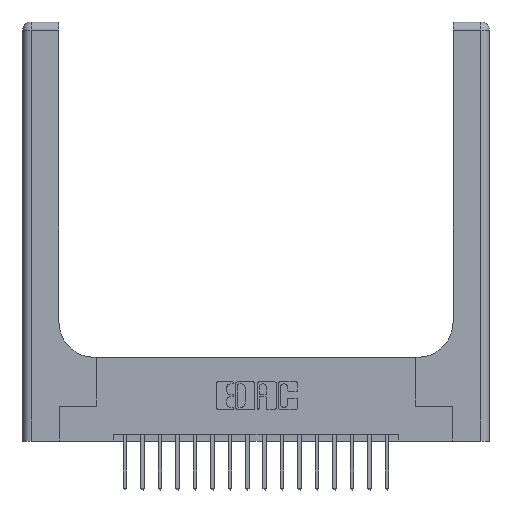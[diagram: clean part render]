
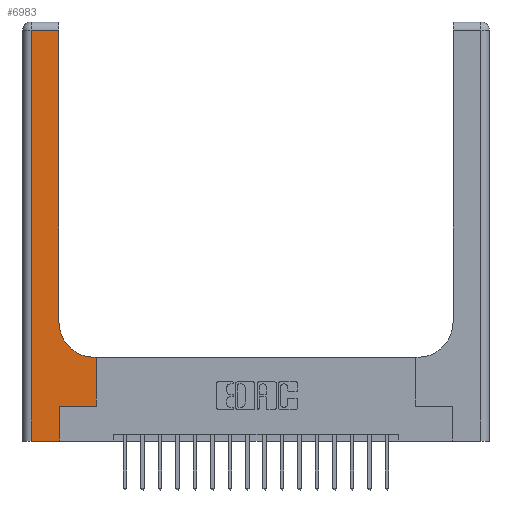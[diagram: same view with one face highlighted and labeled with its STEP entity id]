
A CAD part, top view. The second image highlights one B-rep face of the part: STEP entity #6983.
In plain terms, the highlighted planar face has unit normal (0, 0, 1).
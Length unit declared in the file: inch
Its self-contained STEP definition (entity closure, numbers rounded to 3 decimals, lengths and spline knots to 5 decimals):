
#65 = CARTESIAN_POINT ( 'NONE',  ( 0.26, 3., 0.37 ) ) ;
#98 = CARTESIAN_POINT ( 'NONE',  ( 0., 0., 0.37 ) ) ;
#191 = FACE_OUTER_BOUND ( 'NONE', #6634, .T. ) ;
#386 = CIRCLE ( 'NONE', #13804, 0.25 ) ;
#973 = VERTEX_POINT ( 'NONE', #6647 ) ;
#1305 = LINE ( 'NONE', #98, #8754 ) ;
#1519 = DIRECTION ( 'NONE',  ( 1., 0., 0. ) ) ;
#1708 = EDGE_CURVE ( 'NONE', #2682, #4155, #1305, .T. ) ;
#2682 = VERTEX_POINT ( 'NONE', #3264 ) ;
#2894 = CARTESIAN_POINT ( 'NONE',  ( 0.06, 3., 0.37 ) ) ;
#3031 = EDGE_CURVE ( 'NONE', #9360, #16881, #8223, .T. ) ;
#3187 = ORIENTED_EDGE ( 'NONE', *, *, #3360, .T. ) ;
#3260 = DIRECTION ( 'NONE',  ( 0., 0., -1. ) ) ;
#3264 = CARTESIAN_POINT ( 'NONE',  ( 0.06, 0., 0.37 ) ) ;
#3360 = EDGE_CURVE ( 'NONE', #17764, #8824, #12852, .T. ) ;
#3562 = VECTOR ( 'NONE', #6633, 39.37008 ) ;
#3802 = DIRECTION ( 'NONE',  ( 0., 1., 0. ) ) ;
#4155 = VERTEX_POINT ( 'NONE', #12005 ) ;
#4251 = DIRECTION ( 'NONE',  ( 0., 1., 0. ) ) ;
#4447 = EDGE_CURVE ( 'NONE', #4657, #17764, #12555, .T. ) ;
#4657 = VERTEX_POINT ( 'NONE', #13719 ) ;
#4870 = CARTESIAN_POINT ( 'NONE',  ( 0.51, 0.6, 0.37 ) ) ;
#4910 = DIRECTION ( 'NONE',  ( 0., 0., -1. ) ) ;
#5095 = LINE ( 'NONE', #8159, #12071 ) ;
#5936 = DIRECTION ( 'NONE',  ( 0., -1., 0. ) ) ;
#6104 = ORIENTED_EDGE ( 'NONE', *, *, #14994, .T. ) ;
#6308 = VERTEX_POINT ( 'NONE', #14318 ) ;
#6425 = CARTESIAN_POINT ( 'NONE',  ( 0.26, 2.94, 0.37 ) ) ;
#6633 = DIRECTION ( 'NONE',  ( -1., 0., 0. ) ) ;
#6634 = EDGE_LOOP ( 'NONE', ( #16386, #18016, #6104, #8862, #9578, #8550, #11908, #3187, #15459 ) ) ;
#6647 = CARTESIAN_POINT ( 'NONE',  ( 0.06, 2.94, 0.37 ) ) ;
#6983 = ADVANCED_FACE ( 'NONE', ( #191 ), #16472, .F. ) ;
#7491 = LINE ( 'NONE', #17664, #16979 ) ;
#7697 = DIRECTION ( 'NONE',  ( 0., 1., 0. ) ) ;
#8159 = CARTESIAN_POINT ( 'NONE',  ( 0.265, 0., 0.37 ) ) ;
#8223 = LINE ( 'NONE', #65, #11020 ) ;
#8550 = ORIENTED_EDGE ( 'NONE', *, *, #14991, .T. ) ;
#8754 = VECTOR ( 'NONE', #17756, 39.37008 ) ;
#8824 = VERTEX_POINT ( 'NONE', #4870 ) ;
#8862 = ORIENTED_EDGE ( 'NONE', *, *, #1708, .T. ) ;
#9360 = VERTEX_POINT ( 'NONE', #9566 ) ;
#9566 = CARTESIAN_POINT ( 'NONE',  ( 0.26, 0.85, 0.37 ) ) ;
#9578 = ORIENTED_EDGE ( 'NONE', *, *, #16562, .T. ) ;
#10056 = VECTOR ( 'NONE', #5936, 39.37008 ) ;
#10480 = VECTOR ( 'NONE', #4251, 39.37008 ) ;
#11020 = VECTOR ( 'NONE', #7697, 39.37008 ) ;
#11908 = ORIENTED_EDGE ( 'NONE', *, *, #4447, .T. ) ;
#12005 = CARTESIAN_POINT ( 'NONE',  ( 0.265, 0., 0.37 ) ) ;
#12071 = VECTOR ( 'NONE', #3802, 39.37008 ) ;
#12253 = CARTESIAN_POINT ( 'NONE',  ( 0.51, 0.85, 0.37 ) ) ;
#12555 = LINE ( 'NONE', #13158, #10480 ) ;
#12748 = VECTOR ( 'NONE', #18026, 39.37008 ) ;
#12831 = LINE ( 'NONE', #2894, #10056 ) ;
#12852 = LINE ( 'NONE', #15568, #3562 ) ;
#13001 = EDGE_CURVE ( 'NONE', #8824, #9360, #386, .T. ) ;
#13141 = AXIS2_PLACEMENT_3D ( 'NONE', #16544, #3260, #18029 ) ;
#13158 = CARTESIAN_POINT ( 'NONE',  ( 0.528, 0.25, 0.37 ) ) ;
#13621 = CARTESIAN_POINT ( 'NONE',  ( 0., 2.94, 0.37 ) ) ;
#13719 = CARTESIAN_POINT ( 'NONE',  ( 0.528, 0.25, 0.37 ) ) ;
#13804 = AXIS2_PLACEMENT_3D ( 'NONE', #12253, #4910, #13858 ) ;
#13858 = DIRECTION ( 'NONE',  ( 1., 0., 0. ) ) ;
#13966 = CARTESIAN_POINT ( 'NONE',  ( 0.528, 0.6, 0.37 ) ) ;
#14318 = CARTESIAN_POINT ( 'NONE',  ( 0.265, 0.25, 0.37 ) ) ;
#14598 = LINE ( 'NONE', #13621, #12748 ) ;
#14991 = EDGE_CURVE ( 'NONE', #6308, #4657, #7491, .T. ) ;
#14994 = EDGE_CURVE ( 'NONE', #973, #2682, #12831, .T. ) ;
#15459 = ORIENTED_EDGE ( 'NONE', *, *, #13001, .T. ) ;
#15568 = CARTESIAN_POINT ( 'NONE',  ( 0.26, 0.6, 0.37 ) ) ;
#16386 = ORIENTED_EDGE ( 'NONE', *, *, #3031, .T. ) ;
#16472 = PLANE ( 'NONE',  #13141 ) ;
#16544 = CARTESIAN_POINT ( 'NONE',  ( 0., 3., 0.37 ) ) ;
#16562 = EDGE_CURVE ( 'NONE', #4155, #6308, #5095, .T. ) ;
#16881 = VERTEX_POINT ( 'NONE', #6425 ) ;
#16900 = EDGE_CURVE ( 'NONE', #16881, #973, #14598, .T. ) ;
#16979 = VECTOR ( 'NONE', #1519, 39.37008 ) ;
#17664 = CARTESIAN_POINT ( 'NONE',  ( 0.265, 0.25, 0.37 ) ) ;
#17756 = DIRECTION ( 'NONE',  ( 1., 0., 0. ) ) ;
#17764 = VERTEX_POINT ( 'NONE', #13966 ) ;
#18016 = ORIENTED_EDGE ( 'NONE', *, *, #16900, .T. ) ;
#18026 = DIRECTION ( 'NONE',  ( -1., 0., 0. ) ) ;
#18029 = DIRECTION ( 'NONE',  ( -1., 0., 0. ) ) ;
